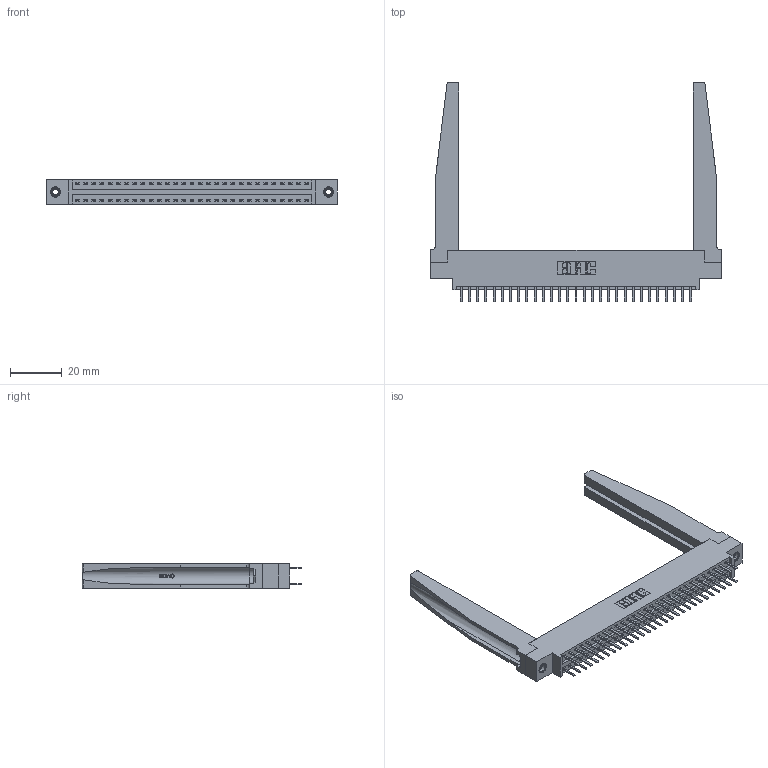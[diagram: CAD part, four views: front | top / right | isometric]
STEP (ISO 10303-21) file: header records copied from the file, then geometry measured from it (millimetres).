
FILE_DESCRIPTION (( 'STEP AP203' ), '1' );
FILE_NAME ('346-058-520-878.STEP', '2022-05-21T07:42:54', ( '' ), ( '' ), 'SwSTEP 2.0', 'SolidWorks 2020', '' );
FILE_SCHEMA (( 'CONFIG_CONTROL_DESIGN' ));
Length unit declared in the file: inch
Products named in the file (5): 346-220-078_345-220-078; 345-250-001_345-250-001-102; 346-058-520-878; 346 Part_0.170 Offset - 0.156 Dia-TH; 345-292-001_345-293-120
Assembly tree (63 placements, depth 2):
  346-058-520-878
    346 Part_0.170 Offset - 0.156 Dia-TH
    345-292-001_345-293-120  x58
    346-220-078_345-220-078  x2
    345-250-001_345-250-001-102  x2
Bounding box: 112.65 x 85.29 x 9.4 mm (x, y, z)
Volume: 17594.4 mm3; surface area: 21175.5 mm2
Topology: 63 solids, 63 shells, 3622 faces, 10439 edges, 6794 vertices
Faces by surface type: plane 2382, cylinder 1188, bspline 36, cone 12, torus 4
Entity records: 26086 total; most frequent: CARTESIAN_POINT 5273, ORIENTED_EDGE 4082, DIRECTION 3671, EDGE_CURVE 2041, VECTOR 1695, LINE 1695, VERTEX_POINT 1352, AXIS2_PLACEMENT_3D 988
